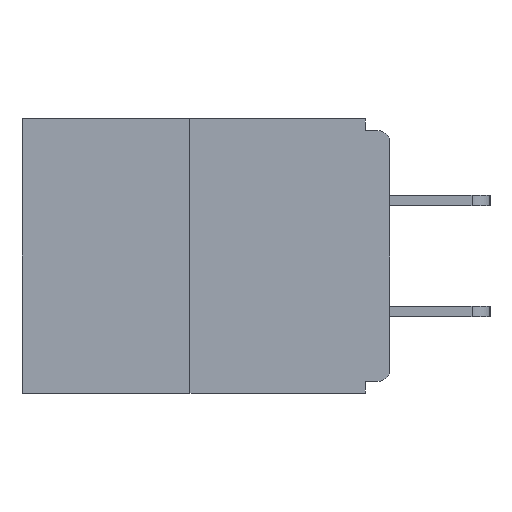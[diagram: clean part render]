
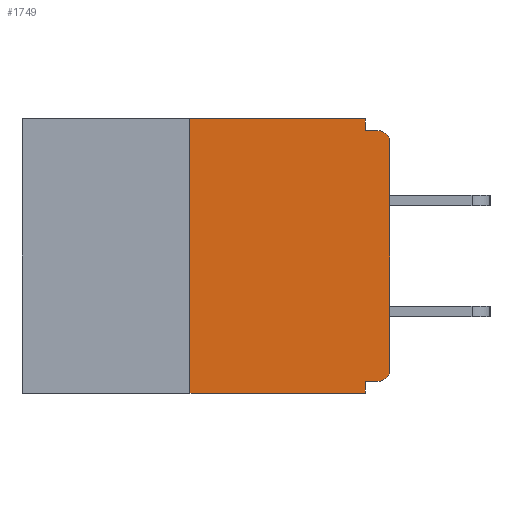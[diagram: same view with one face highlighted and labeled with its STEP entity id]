
A CAD part, left-side view. The second image highlights one B-rep face of the part: STEP entity #1749.
In plain terms, the highlighted planar face has unit normal (-1, 0, 0).
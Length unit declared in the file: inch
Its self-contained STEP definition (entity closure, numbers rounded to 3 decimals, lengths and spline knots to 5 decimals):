
#33 = EDGE_CURVE ( 'NONE', #13506, #18317, #9807, .T. ) ;
#334 = CARTESIAN_POINT ( 'NONE',  ( 0., 0.031, 0. ) ) ;
#516 = PLANE ( 'NONE',  #10877 ) ;
#957 = LINE ( 'NONE', #3605, #3859 ) ;
#1749 = ADVANCED_FACE ( 'NONE', ( #16899 ), #516, .F. ) ;
#2130 = VECTOR ( 'NONE', #12186, 39.37008 ) ;
#2519 = DIRECTION ( 'NONE',  ( -1., 0., 0. ) ) ;
#3283 = ORIENTED_EDGE ( 'NONE', *, *, #16436, .T. ) ;
#3431 = CARTESIAN_POINT ( 'NONE',  ( 0., 0.031, -0.328 ) ) ;
#3438 = VERTEX_POINT ( 'NONE', #14077 ) ;
#3605 = CARTESIAN_POINT ( 'NONE',  ( 0., 0., 0. ) ) ;
#3631 = CARTESIAN_POINT ( 'NONE',  ( 0., 0.46, 0. ) ) ;
#3859 = VECTOR ( 'NONE', #12600, 39.37008 ) ;
#4271 = ORIENTED_EDGE ( 'NONE', *, *, #11121, .T. ) ;
#4460 = EDGE_LOOP ( 'NONE', ( #6765, #19212, #3283, #16725, #14127, #18131, #4271, #14696, #17151, #18853 ) ) ;
#4474 = VERTEX_POINT ( 'NONE', #18814 ) ;
#4842 = LINE ( 'NONE', #12022, #6035 ) ;
#5049 = DIRECTION ( 'NONE',  ( 0., 0., -1. ) ) ;
#5293 = LINE ( 'NONE', #17481, #14349 ) ;
#5702 = EDGE_CURVE ( 'NONE', #7573, #16052, #8509, .T. ) ;
#6019 = CARTESIAN_POINT ( 'NONE',  ( 0., 0.031, -0.343 ) ) ;
#6035 = VECTOR ( 'NONE', #12093, 39.37008 ) ;
#6499 = AXIS2_PLACEMENT_3D ( 'NONE', #11524, #17817, #13111 ) ;
#6765 = ORIENTED_EDGE ( 'NONE', *, *, #13372, .F. ) ;
#6830 = DIRECTION ( 'NONE',  ( 0., 0., 1. ) ) ;
#6889 = EDGE_CURVE ( 'NONE', #7550, #4474, #7897, .T. ) ;
#7158 = EDGE_CURVE ( 'NONE', #3438, #14731, #5293, .T. ) ;
#7240 = AXIS2_PLACEMENT_3D ( 'NONE', #14712, #2519, #19326 ) ;
#7550 = VERTEX_POINT ( 'NONE', #19798 ) ;
#7573 = VERTEX_POINT ( 'NONE', #16763 ) ;
#7897 = CIRCLE ( 'NONE', #6499, 0.015 ) ;
#8227 = VERTEX_POINT ( 'NONE', #9681 ) ;
#8509 = CIRCLE ( 'NONE', #7240, 0.015 ) ;
#8794 = DIRECTION ( 'NONE',  ( 0., 1., 0. ) ) ;
#9145 = VERTEX_POINT ( 'NONE', #15253 ) ;
#9193 = EDGE_CURVE ( 'NONE', #8227, #16052, #13218, .T. ) ;
#9681 = CARTESIAN_POINT ( 'NONE',  ( 0., 0.031, -0.015 ) ) ;
#9807 = LINE ( 'NONE', #6019, #2130 ) ;
#10049 = LINE ( 'NONE', #16304, #10506 ) ;
#10506 = VECTOR ( 'NONE', #8794, 39.37008 ) ;
#10759 = DIRECTION ( 'NONE',  ( 0., -1., 0. ) ) ;
#10877 = AXIS2_PLACEMENT_3D ( 'NONE', #3631, #12703, #5049 ) ;
#11121 = EDGE_CURVE ( 'NONE', #4474, #7573, #957, .T. ) ;
#11440 = EDGE_CURVE ( 'NONE', #7550, #13506, #10049, .T. ) ;
#11524 = CARTESIAN_POINT ( 'NONE',  ( 0., 0.015, -0.313 ) ) ;
#12022 = CARTESIAN_POINT ( 'NONE',  ( 0., 0.46, 0. ) ) ;
#12093 = DIRECTION ( 'NONE',  ( 0., -1., 0. ) ) ;
#12186 = DIRECTION ( 'NONE',  ( 0., 0., -1. ) ) ;
#12599 = VECTOR ( 'NONE', #18357, 39.37008 ) ;
#12600 = DIRECTION ( 'NONE',  ( 0., 0., 1. ) ) ;
#12703 = DIRECTION ( 'NONE',  ( 1., 0., 0. ) ) ;
#12945 = CARTESIAN_POINT ( 'NONE',  ( 0., 0.015, -0.015 ) ) ;
#13111 = DIRECTION ( 'NONE',  ( 0., 0., -1. ) ) ;
#13218 = LINE ( 'NONE', #16867, #19677 ) ;
#13281 = CARTESIAN_POINT ( 'NONE',  ( 0., 0.25, 0. ) ) ;
#13372 = EDGE_CURVE ( 'NONE', #14731, #9145, #4842, .T. ) ;
#13506 = VERTEX_POINT ( 'NONE', #3431 ) ;
#14077 = CARTESIAN_POINT ( 'NONE',  ( 0., 0.25, -0.343 ) ) ;
#14127 = ORIENTED_EDGE ( 'NONE', *, *, #11440, .F. ) ;
#14257 = DIRECTION ( 'NONE',  ( 0., 0., -1. ) ) ;
#14349 = VECTOR ( 'NONE', #6830, 39.37008 ) ;
#14552 = VECTOR ( 'NONE', #14257, 39.37008 ) ;
#14696 = ORIENTED_EDGE ( 'NONE', *, *, #5702, .T. ) ;
#14712 = CARTESIAN_POINT ( 'NONE',  ( 0., 0.015, -0.03 ) ) ;
#14731 = VERTEX_POINT ( 'NONE', #13281 ) ;
#15253 = CARTESIAN_POINT ( 'NONE',  ( 0., 0.031, 0. ) ) ;
#16052 = VERTEX_POINT ( 'NONE', #12945 ) ;
#16304 = CARTESIAN_POINT ( 'NONE',  ( 0., 0., -0.328 ) ) ;
#16436 = EDGE_CURVE ( 'NONE', #3438, #18317, #17676, .T. ) ;
#16595 = EDGE_CURVE ( 'NONE', #9145, #8227, #17188, .T. ) ;
#16725 = ORIENTED_EDGE ( 'NONE', *, *, #33, .F. ) ;
#16763 = CARTESIAN_POINT ( 'NONE',  ( 0., 0., -0.03 ) ) ;
#16867 = CARTESIAN_POINT ( 'NONE',  ( 0., 0., -0.015 ) ) ;
#16899 = FACE_OUTER_BOUND ( 'NONE', #4460, .T. ) ;
#17151 = ORIENTED_EDGE ( 'NONE', *, *, #9193, .F. ) ;
#17188 = LINE ( 'NONE', #334, #14552 ) ;
#17481 = CARTESIAN_POINT ( 'NONE',  ( 0., 0.25, 0. ) ) ;
#17676 = LINE ( 'NONE', #18434, #12599 ) ;
#17817 = DIRECTION ( 'NONE',  ( -1., 0., 0. ) ) ;
#18131 = ORIENTED_EDGE ( 'NONE', *, *, #6889, .T. ) ;
#18317 = VERTEX_POINT ( 'NONE', #18949 ) ;
#18357 = DIRECTION ( 'NONE',  ( 0., -1., 0. ) ) ;
#18434 = CARTESIAN_POINT ( 'NONE',  ( 0., 0.46, -0.343 ) ) ;
#18814 = CARTESIAN_POINT ( 'NONE',  ( 0., 0., -0.313 ) ) ;
#18853 = ORIENTED_EDGE ( 'NONE', *, *, #16595, .F. ) ;
#18949 = CARTESIAN_POINT ( 'NONE',  ( 0., 0.031, -0.343 ) ) ;
#19212 = ORIENTED_EDGE ( 'NONE', *, *, #7158, .F. ) ;
#19326 = DIRECTION ( 'NONE',  ( 0., 0., -1. ) ) ;
#19677 = VECTOR ( 'NONE', #10759, 39.37008 ) ;
#19798 = CARTESIAN_POINT ( 'NONE',  ( 0., 0.015, -0.328 ) ) ;
